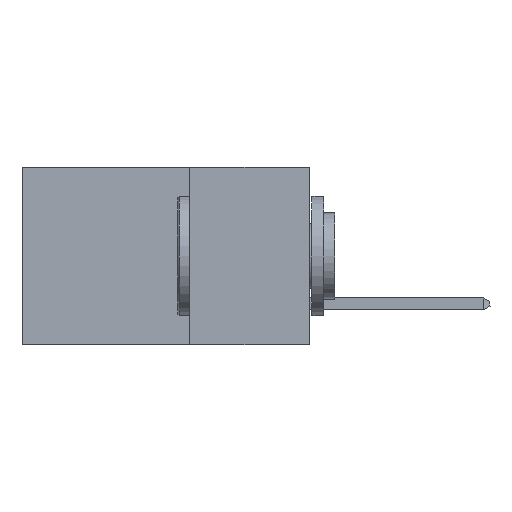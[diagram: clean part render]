
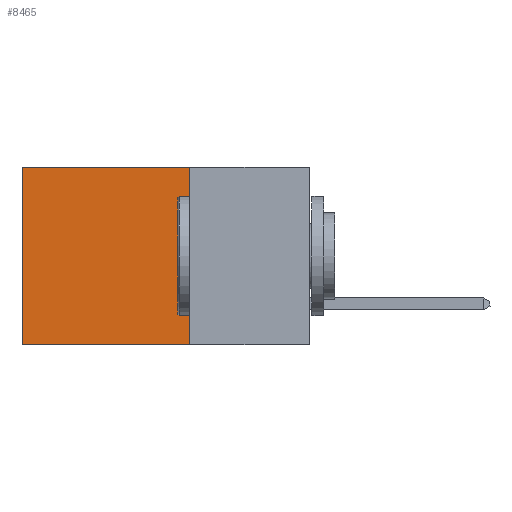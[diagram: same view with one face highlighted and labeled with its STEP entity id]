
A CAD part, left-side view. The second image highlights one B-rep face of the part: STEP entity #8465.
In plain terms, the highlighted planar face has unit normal (-1, 0, 0).
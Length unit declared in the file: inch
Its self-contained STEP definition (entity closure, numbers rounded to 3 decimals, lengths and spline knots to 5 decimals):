
#386 = LINE ( 'NONE', #3344, #17911 ) ;
#1291 = CARTESIAN_POINT ( 'NONE',  ( 0.2875, 0.25, 0. ) ) ;
#1561 = CARTESIAN_POINT ( 'NONE',  ( 0.2875, 0.25, -0.37 ) ) ;
#2064 = VECTOR ( 'NONE', #3027, 39.37008 ) ;
#2421 = AXIS2_PLACEMENT_3D ( 'NONE', #16659, #18251, #8356 ) ;
#2774 = ORIENTED_EDGE ( 'NONE', *, *, #6127, .F. ) ;
#3027 = DIRECTION ( 'NONE',  ( 0., 1., 0. ) ) ;
#3344 = CARTESIAN_POINT ( 'NONE',  ( 0.2875, 0.25, 0. ) ) ;
#3377 = FACE_OUTER_BOUND ( 'NONE', #17720, .T. ) ;
#3395 = CARTESIAN_POINT ( 'NONE',  ( 0.2875, 0.6, -0.37 ) ) ;
#3867 = VERTEX_POINT ( 'NONE', #12079 ) ;
#3999 = CARTESIAN_POINT ( 'NONE',  ( 0.2875, 0.6, 0. ) ) ;
#6127 = EDGE_CURVE ( 'NONE', #11060, #11159, #14796, .T. ) ;
#7258 = VERTEX_POINT ( 'NONE', #1291 ) ;
#7627 = EDGE_CURVE ( 'NONE', #3867, #11159, #15429, .T. ) ;
#7896 = EDGE_CURVE ( 'NONE', #7258, #3867, #11271, .T. ) ;
#8356 = DIRECTION ( 'NONE',  ( 0., 0., -1. ) ) ;
#8465 = ADVANCED_FACE ( 'NONE', ( #3377 ), #13368, .F. ) ;
#8590 = ORIENTED_EDGE ( 'NONE', *, *, #9072, .F. ) ;
#9072 = EDGE_CURVE ( 'NONE', #7258, #11060, #386, .T. ) ;
#10023 = CARTESIAN_POINT ( 'NONE',  ( 0.2875, 0.25, -0.37 ) ) ;
#11005 = VECTOR ( 'NONE', #14258, 39.37008 ) ;
#11060 = VERTEX_POINT ( 'NONE', #10023 ) ;
#11159 = VERTEX_POINT ( 'NONE', #3395 ) ;
#11271 = LINE ( 'NONE', #14997, #2064 ) ;
#11941 = DIRECTION ( 'NONE',  ( 0., 1., 0. ) ) ;
#12079 = CARTESIAN_POINT ( 'NONE',  ( 0.2875, 0.6, 0. ) ) ;
#12470 = ORIENTED_EDGE ( 'NONE', *, *, #7896, .T. ) ;
#13368 = PLANE ( 'NONE',  #2421 ) ;
#13626 = DIRECTION ( 'NONE',  ( 0., 0., -1. ) ) ;
#14251 = VECTOR ( 'NONE', #11941, 39.37008 ) ;
#14258 = DIRECTION ( 'NONE',  ( 0., 0., -1. ) ) ;
#14406 = ORIENTED_EDGE ( 'NONE', *, *, #7627, .T. ) ;
#14796 = LINE ( 'NONE', #1561, #14251 ) ;
#14997 = CARTESIAN_POINT ( 'NONE',  ( 0.2875, 0.25, 0. ) ) ;
#15429 = LINE ( 'NONE', #3999, #11005 ) ;
#16659 = CARTESIAN_POINT ( 'NONE',  ( 0.2875, 0.25, 0. ) ) ;
#17720 = EDGE_LOOP ( 'NONE', ( #14406, #2774, #8590, #12470 ) ) ;
#17911 = VECTOR ( 'NONE', #13626, 39.37008 ) ;
#18251 = DIRECTION ( 'NONE',  ( 1., 0., 0. ) ) ;
